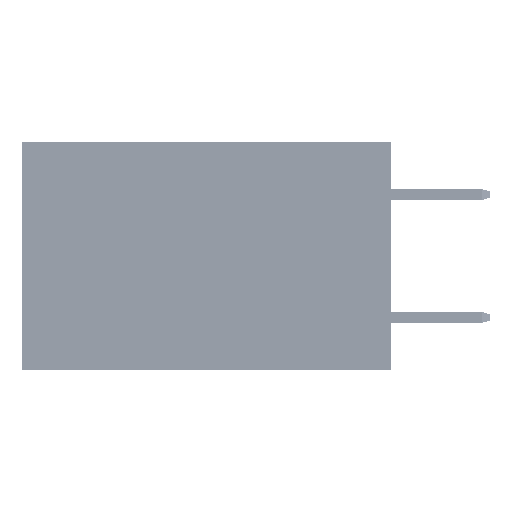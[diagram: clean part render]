
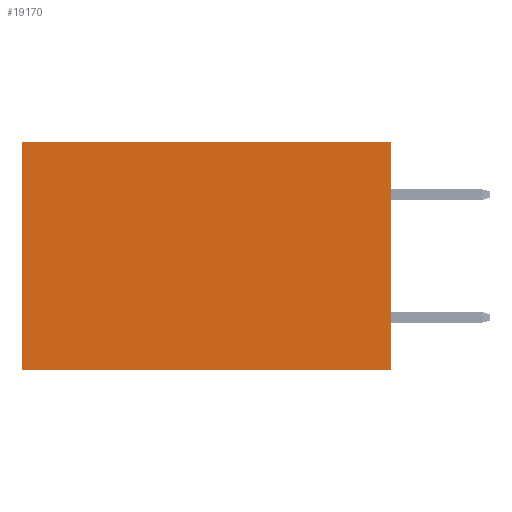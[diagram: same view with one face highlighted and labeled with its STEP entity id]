
A CAD part, left-side view. The second image highlights one B-rep face of the part: STEP entity #19170.
In plain terms, the highlighted planar face has unit normal (-1, 0, 0).
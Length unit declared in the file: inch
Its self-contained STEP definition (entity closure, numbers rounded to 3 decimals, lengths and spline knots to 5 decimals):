
#68 = EDGE_CURVE ( 'NONE', #17417, #7175, #46805, .T. ) ;
#2816 = CARTESIAN_POINT ( 'NONE',  ( 0.2875, 0.6, 0. ) ) ;
#3557 = EDGE_CURVE ( 'NONE', #17417, #19913, #33035, .T. ) ;
#4778 = CARTESIAN_POINT ( 'NONE',  ( 0.2875, 0., 0. ) ) ;
#7175 = VERTEX_POINT ( 'NONE', #2816 ) ;
#8726 = FACE_OUTER_BOUND ( 'NONE', #42287, .T. ) ;
#9690 = DIRECTION ( 'NONE',  ( 0., 0., -1. ) ) ;
#11600 = PLANE ( 'NONE',  #35442 ) ;
#12774 = DIRECTION ( 'NONE',  ( 0., 1., 0. ) ) ;
#13683 = EDGE_CURVE ( 'NONE', #7175, #42763, #26786, .T. ) ;
#15775 = DIRECTION ( 'NONE',  ( 0., 0., -1. ) ) ;
#17417 = VERTEX_POINT ( 'NONE', #4778 ) ;
#19170 = ADVANCED_FACE ( 'NONE', ( #8726 ), #11600, .F. ) ;
#19640 = CARTESIAN_POINT ( 'NONE',  ( 0.2875, 0., 0. ) ) ;
#19903 = ORIENTED_EDGE ( 'NONE', *, *, #3557, .F. ) ;
#19913 = VERTEX_POINT ( 'NONE', #31722 ) ;
#23749 = VECTOR ( 'NONE', #30919, 39.37008 ) ;
#26786 = LINE ( 'NONE', #33515, #38590 ) ;
#27559 = CARTESIAN_POINT ( 'NONE',  ( 0.2875, 0.6, -0.37 ) ) ;
#29309 = CARTESIAN_POINT ( 'NONE',  ( 0.2875, 0., 0. ) ) ;
#30919 = DIRECTION ( 'NONE',  ( 0., 0., -1. ) ) ;
#31722 = CARTESIAN_POINT ( 'NONE',  ( 0.2875, 0., -0.37 ) ) ;
#32392 = VECTOR ( 'NONE', #47726, 39.37008 ) ;
#33035 = LINE ( 'NONE', #46730, #23749 ) ;
#33515 = CARTESIAN_POINT ( 'NONE',  ( 0.2875, 0.6, 0. ) ) ;
#33735 = VECTOR ( 'NONE', #12774, 39.37008 ) ;
#35442 = AXIS2_PLACEMENT_3D ( 'NONE', #19640, #39591, #15775 ) ;
#35732 = CARTESIAN_POINT ( 'NONE',  ( 0.2875, 0., -0.37 ) ) ;
#36684 = EDGE_CURVE ( 'NONE', #19913, #42763, #42972, .T. ) ;
#37687 = ORIENTED_EDGE ( 'NONE', *, *, #13683, .T. ) ;
#38590 = VECTOR ( 'NONE', #9690, 39.37008 ) ;
#39591 = DIRECTION ( 'NONE',  ( 1., 0., 0. ) ) ;
#42287 = EDGE_LOOP ( 'NONE', ( #37687, #50686, #19903, #44018 ) ) ;
#42763 = VERTEX_POINT ( 'NONE', #27559 ) ;
#42972 = LINE ( 'NONE', #35732, #32392 ) ;
#44018 = ORIENTED_EDGE ( 'NONE', *, *, #68, .T. ) ;
#46730 = CARTESIAN_POINT ( 'NONE',  ( 0.2875, 0., 0. ) ) ;
#46805 = LINE ( 'NONE', #29309, #33735 ) ;
#47726 = DIRECTION ( 'NONE',  ( 0., 1., 0. ) ) ;
#50686 = ORIENTED_EDGE ( 'NONE', *, *, #36684, .F. ) ;
